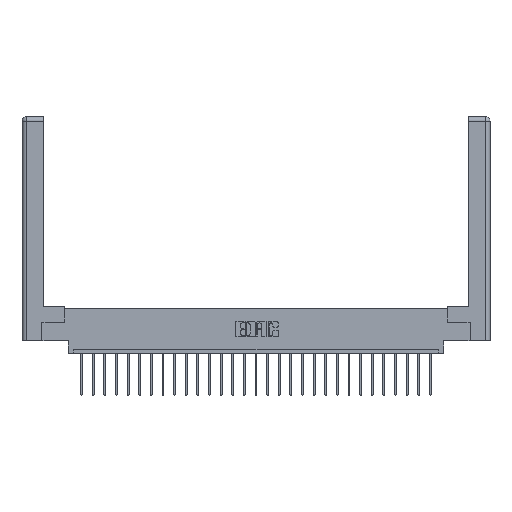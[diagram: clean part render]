
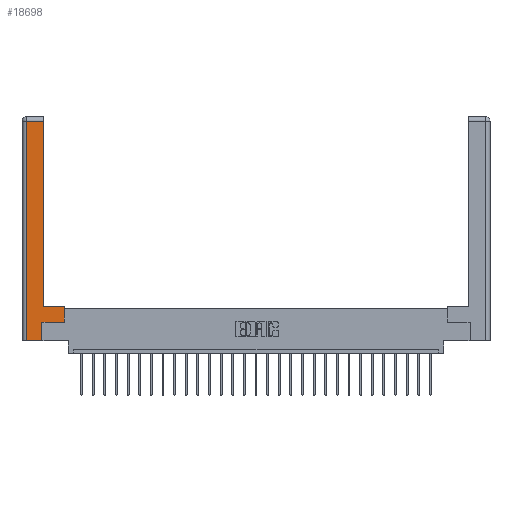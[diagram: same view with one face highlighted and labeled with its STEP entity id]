
A CAD part, top view. The second image highlights one B-rep face of the part: STEP entity #18698.
In plain terms, the highlighted planar face has unit normal (0, 0, 1).
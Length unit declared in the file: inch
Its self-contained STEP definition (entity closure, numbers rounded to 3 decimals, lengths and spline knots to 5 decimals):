
#93 = LINE ( 'NONE', #13108, #18210 ) ;
#609 = VECTOR ( 'NONE', #26186, 39.37008 ) ;
#1009 = CARTESIAN_POINT ( 'NONE',  ( 0., 0., 0. ) ) ;
#1198 = DIRECTION ( 'NONE',  ( -1., 0., 0. ) ) ;
#3507 = CARTESIAN_POINT ( 'NONE',  ( 0.295, 0.45, 0. ) ) ;
#3594 = LINE ( 'NONE', #16896, #20375 ) ;
#3834 = DIRECTION ( 'NONE',  ( 0., -1., 0. ) ) ;
#5004 = CARTESIAN_POINT ( 'NONE',  ( 0.565, 0.45, 0. ) ) ;
#5042 = DIRECTION ( 'NONE',  ( 1., 0., 0. ) ) ;
#5280 = ORIENTED_EDGE ( 'NONE', *, *, #26726, .T. ) ;
#5310 = DIRECTION ( 'NONE',  ( 0., 0., -1. ) ) ;
#5746 = EDGE_CURVE ( 'NONE', #8235, #9969, #24242, .T. ) ;
#6336 = ORIENTED_EDGE ( 'NONE', *, *, #24173, .T. ) ;
#6407 = CARTESIAN_POINT ( 'NONE',  ( 0.0615, 2.94, 0. ) ) ;
#6635 = CARTESIAN_POINT ( 'NONE',  ( 0.565, 0.245, 0. ) ) ;
#6684 = EDGE_CURVE ( 'NONE', #23975, #10770, #20791, .T. ) ;
#6838 = CARTESIAN_POINT ( 'NONE',  ( 0.295, 2.94, 0. ) ) ;
#7008 = VECTOR ( 'NONE', #3834, 39.37008 ) ;
#7625 = VECTOR ( 'NONE', #23800, 39.37008 ) ;
#8235 = VERTEX_POINT ( 'NONE', #25479 ) ;
#8786 = CARTESIAN_POINT ( 'NONE',  ( 0.565, 0.45, 0. ) ) ;
#9235 = CARTESIAN_POINT ( 'NONE',  ( 0.265, 0.245, 0. ) ) ;
#9969 = VERTEX_POINT ( 'NONE', #6635 ) ;
#10770 = VERTEX_POINT ( 'NONE', #3507 ) ;
#11480 = CARTESIAN_POINT ( 'NONE',  ( 0.295, 0.45, 0. ) ) ;
#12275 = CARTESIAN_POINT ( 'NONE',  ( 0.0615, 0., 0. ) ) ;
#12310 = ORIENTED_EDGE ( 'NONE', *, *, #24130, .T. ) ;
#12449 = ORIENTED_EDGE ( 'NONE', *, *, #21838, .T. ) ;
#12477 = DIRECTION ( 'NONE',  ( 0., 1., 0. ) ) ;
#12556 = ORIENTED_EDGE ( 'NONE', *, *, #23970, .T. ) ;
#12583 = LINE ( 'NONE', #12275, #7008 ) ;
#12844 = LINE ( 'NONE', #6407, #21379 ) ;
#12960 = VECTOR ( 'NONE', #5042, 39.37008 ) ;
#13108 = CARTESIAN_POINT ( 'NONE',  ( 0.265, 0., 0. ) ) ;
#13433 = VERTEX_POINT ( 'NONE', #26367 ) ;
#13868 = LINE ( 'NONE', #5004, #7625 ) ;
#15141 = DIRECTION ( 'NONE',  ( -1., 0., 0. ) ) ;
#15234 = DIRECTION ( 'NONE',  ( 1., 0., 0. ) ) ;
#16786 = ORIENTED_EDGE ( 'NONE', *, *, #25213, .T. ) ;
#16896 = CARTESIAN_POINT ( 'NONE',  ( 0.295, 3., 0. ) ) ;
#17704 = VERTEX_POINT ( 'NONE', #6838 ) ;
#18067 = EDGE_LOOP ( 'NONE', ( #5280, #12556, #6336, #12310, #12449, #27211, #16786, #24977 ) ) ;
#18210 = VECTOR ( 'NONE', #15234, 39.37008 ) ;
#18698 = ADVANCED_FACE ( 'NONE', ( #22851 ), #26232, .F. ) ;
#19573 = CARTESIAN_POINT ( 'NONE',  ( 0.565, 0.245, 0. ) ) ;
#20375 = VECTOR ( 'NONE', #12477, 39.37008 ) ;
#20791 = LINE ( 'NONE', #11480, #23432 ) ;
#21379 = VECTOR ( 'NONE', #15141, 39.37008 ) ;
#21407 = CARTESIAN_POINT ( 'NONE',  ( 0.265, 0., 0. ) ) ;
#21716 = CARTESIAN_POINT ( 'NONE',  ( 0.0615, 0., 0. ) ) ;
#21838 = EDGE_CURVE ( 'NONE', #26375, #8235, #24312, .T. ) ;
#21898 = DIRECTION ( 'NONE',  ( -1., 0., 0. ) ) ;
#22851 = FACE_OUTER_BOUND ( 'NONE', #18067, .T. ) ;
#23432 = VECTOR ( 'NONE', #21898, 39.37008 ) ;
#23800 = DIRECTION ( 'NONE',  ( 0., 1., 0. ) ) ;
#23970 = EDGE_CURVE ( 'NONE', #17704, #13433, #12844, .T. ) ;
#23975 = VERTEX_POINT ( 'NONE', #8786 ) ;
#24130 = EDGE_CURVE ( 'NONE', #24425, #26375, #93, .T. ) ;
#24173 = EDGE_CURVE ( 'NONE', #13433, #24425, #12583, .T. ) ;
#24199 = AXIS2_PLACEMENT_3D ( 'NONE', #1009, #5310, #1198 ) ;
#24242 = LINE ( 'NONE', #19573, #12960 ) ;
#24312 = LINE ( 'NONE', #9235, #609 ) ;
#24425 = VERTEX_POINT ( 'NONE', #21716 ) ;
#24977 = ORIENTED_EDGE ( 'NONE', *, *, #6684, .T. ) ;
#25213 = EDGE_CURVE ( 'NONE', #9969, #23975, #13868, .T. ) ;
#25479 = CARTESIAN_POINT ( 'NONE',  ( 0.265, 0.245, 0. ) ) ;
#26186 = DIRECTION ( 'NONE',  ( 0., 1., 0. ) ) ;
#26232 = PLANE ( 'NONE',  #24199 ) ;
#26367 = CARTESIAN_POINT ( 'NONE',  ( 0.0615, 2.94, 0. ) ) ;
#26375 = VERTEX_POINT ( 'NONE', #21407 ) ;
#26726 = EDGE_CURVE ( 'NONE', #10770, #17704, #3594, .T. ) ;
#27211 = ORIENTED_EDGE ( 'NONE', *, *, #5746, .T. ) ;
